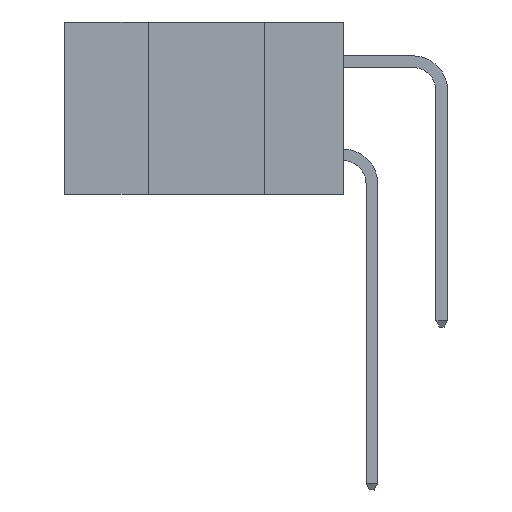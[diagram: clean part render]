
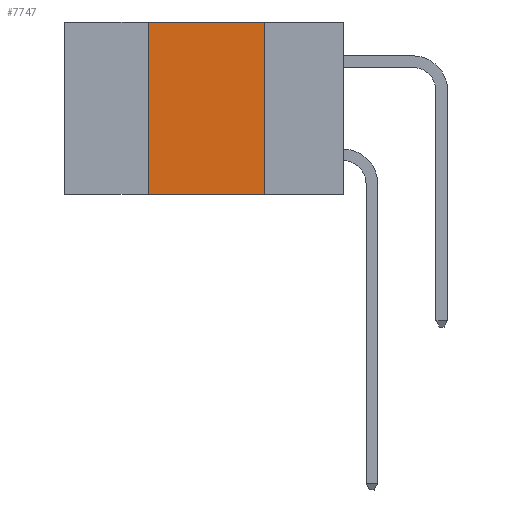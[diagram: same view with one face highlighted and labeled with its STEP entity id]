
A CAD part, left-side view. The second image highlights one B-rep face of the part: STEP entity #7747.
In plain terms, the highlighted planar face has unit normal (-1, 0, 0).
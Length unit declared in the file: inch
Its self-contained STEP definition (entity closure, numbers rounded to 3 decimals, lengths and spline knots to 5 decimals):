
#561 = VERTEX_POINT ( 'NONE', #33019 ) ;
#2734 = LINE ( 'NONE', #29685, #28151 ) ;
#4212 = ORIENTED_EDGE ( 'NONE', *, *, #28241, .T. ) ;
#4746 = VECTOR ( 'NONE', #20372, 39.37008 ) ;
#5857 = VERTEX_POINT ( 'NONE', #11161 ) ;
#6461 = CARTESIAN_POINT ( 'NONE',  ( 0., 0.17, 0. ) ) ;
#7609 = EDGE_CURVE ( 'NONE', #20283, #5857, #17831, .T. ) ;
#7747 = ADVANCED_FACE ( 'NONE', ( #35271 ), #8218, .F. ) ;
#8218 = PLANE ( 'NONE',  #23086 ) ;
#8853 = ORIENTED_EDGE ( 'NONE', *, *, #19795, .F. ) ;
#9415 = CARTESIAN_POINT ( 'NONE',  ( 0., 0.6, -0.37 ) ) ;
#11161 = CARTESIAN_POINT ( 'NONE',  ( 0., 0.17, -0.37 ) ) ;
#13570 = EDGE_CURVE ( 'NONE', #561, #27765, #2734, .T. ) ;
#13726 = DIRECTION ( 'NONE',  ( 1., 0., 0. ) ) ;
#13810 = DIRECTION ( 'NONE',  ( 0., -1., 0. ) ) ;
#14641 = DIRECTION ( 'NONE',  ( 0., 0., -1. ) ) ;
#15338 = CARTESIAN_POINT ( 'NONE',  ( 0., 0.17, 0. ) ) ;
#16490 = EDGE_LOOP ( 'NONE', ( #25835, #8853, #25128, #4212 ) ) ;
#17831 = LINE ( 'NONE', #6461, #19096 ) ;
#19096 = VECTOR ( 'NONE', #14641, 39.37008 ) ;
#19505 = VECTOR ( 'NONE', #13810, 39.37008 ) ;
#19795 = EDGE_CURVE ( 'NONE', #27765, #20283, #24235, .T. ) ;
#20283 = VERTEX_POINT ( 'NONE', #15338 ) ;
#20372 = DIRECTION ( 'NONE',  ( 0., -1., 0. ) ) ;
#23086 = AXIS2_PLACEMENT_3D ( 'NONE', #29714, #13726, #27436 ) ;
#24235 = LINE ( 'NONE', #30031, #19505 ) ;
#25128 = ORIENTED_EDGE ( 'NONE', *, *, #13570, .F. ) ;
#25835 = ORIENTED_EDGE ( 'NONE', *, *, #7609, .F. ) ;
#27436 = DIRECTION ( 'NONE',  ( 0., 0., -1. ) ) ;
#27765 = VERTEX_POINT ( 'NONE', #35004 ) ;
#28151 = VECTOR ( 'NONE', #35052, 39.37008 ) ;
#28241 = EDGE_CURVE ( 'NONE', #561, #5857, #28408, .T. ) ;
#28408 = LINE ( 'NONE', #9415, #4746 ) ;
#29685 = CARTESIAN_POINT ( 'NONE',  ( 0., 0.42, 0. ) ) ;
#29714 = CARTESIAN_POINT ( 'NONE',  ( 0., 0.6, 0. ) ) ;
#30031 = CARTESIAN_POINT ( 'NONE',  ( 0., 0.6, 0. ) ) ;
#33019 = CARTESIAN_POINT ( 'NONE',  ( 0., 0.42, -0.37 ) ) ;
#35004 = CARTESIAN_POINT ( 'NONE',  ( 0., 0.42, 0. ) ) ;
#35052 = DIRECTION ( 'NONE',  ( 0., 0., 1. ) ) ;
#35271 = FACE_OUTER_BOUND ( 'NONE', #16490, .T. ) ;
